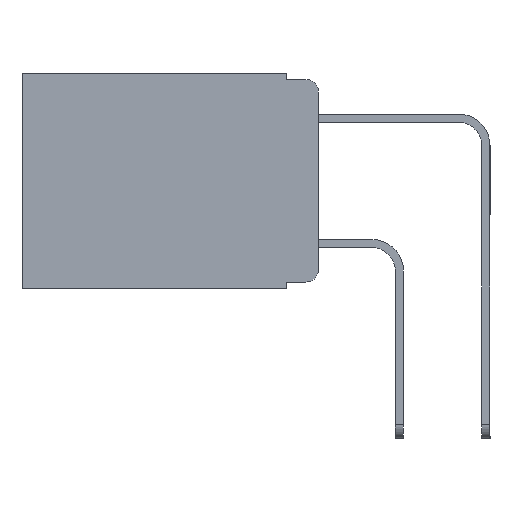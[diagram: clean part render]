
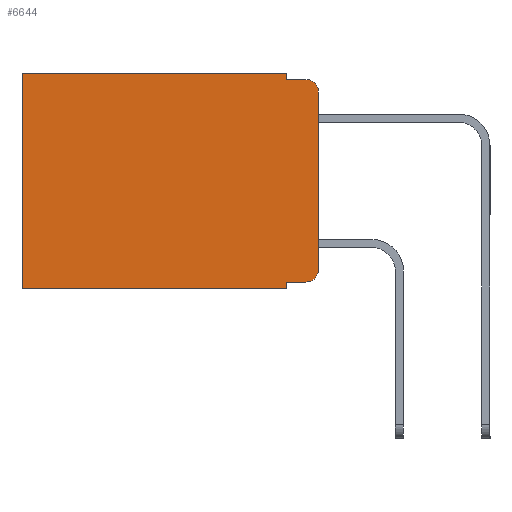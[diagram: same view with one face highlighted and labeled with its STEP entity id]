
A CAD part, left-side view. The second image highlights one B-rep face of the part: STEP entity #6644.
In plain terms, the highlighted planar face has unit normal (-1, 0, 0).
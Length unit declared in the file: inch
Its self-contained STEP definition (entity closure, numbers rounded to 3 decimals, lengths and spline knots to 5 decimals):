
#72 = ORIENTED_EDGE ( 'NONE', *, *, #3603, .T. ) ;
#216 = CARTESIAN_POINT ( 'NONE',  ( 0.298, 0., 0. ) ) ;
#468 = AXIS2_PLACEMENT_3D ( 'NONE', #3854, #10732, #11676 ) ;
#496 = DIRECTION ( 'NONE',  ( 0., 1., 0. ) ) ;
#576 = CARTESIAN_POINT ( 'NONE',  ( 0.298, 0.051, 0. ) ) ;
#677 = CARTESIAN_POINT ( 'NONE',  ( 0.298, 0.051, -0.333 ) ) ;
#688 = AXIS2_PLACEMENT_3D ( 'NONE', #8236, #6756, #6740 ) ;
#906 = CARTESIAN_POINT ( 'NONE',  ( 0.298, 0.02, -0.01 ) ) ;
#927 = CARTESIAN_POINT ( 'NONE',  ( 0.298, 0.473, -0.343 ) ) ;
#1081 = DIRECTION ( 'NONE',  ( 0., 0., -1. ) ) ;
#1325 = ORIENTED_EDGE ( 'NONE', *, *, #8675, .T. ) ;
#1689 = ORIENTED_EDGE ( 'NONE', *, *, #1794, .F. ) ;
#1720 = VERTEX_POINT ( 'NONE', #9600 ) ;
#1772 = EDGE_CURVE ( 'NONE', #12145, #12700, #9270, .T. ) ;
#1794 = EDGE_CURVE ( 'NONE', #6048, #1720, #3552, .T. ) ;
#1948 = DIRECTION ( 'NONE',  ( 0., -1., 0. ) ) ;
#2031 = ORIENTED_EDGE ( 'NONE', *, *, #2812, .F. ) ;
#2391 = VECTOR ( 'NONE', #496, 39.37008 ) ;
#2433 = VECTOR ( 'NONE', #1948, 39.37008 ) ;
#2766 = DIRECTION ( 'NONE',  ( 0., 1., 0. ) ) ;
#2773 = CARTESIAN_POINT ( 'NONE',  ( 0.298, 0.051, 0. ) ) ;
#2812 = EDGE_CURVE ( 'NONE', #8598, #4335, #10800, .T. ) ;
#3003 = FACE_OUTER_BOUND ( 'NONE', #3454, .T. ) ;
#3037 = VECTOR ( 'NONE', #5504, 39.37008 ) ;
#3120 = ORIENTED_EDGE ( 'NONE', *, *, #8449, .T. ) ;
#3154 = VECTOR ( 'NONE', #5846, 39.37008 ) ;
#3243 = VERTEX_POINT ( 'NONE', #927 ) ;
#3283 = VERTEX_POINT ( 'NONE', #9086 ) ;
#3401 = LINE ( 'NONE', #10273, #3037 ) ;
#3454 = EDGE_LOOP ( 'NONE', ( #1689, #1325, #2031, #4684, #8053, #12683, #8339, #10476, #3120, #72 ) ) ;
#3552 = LINE ( 'NONE', #5144, #9555 ) ;
#3603 = EDGE_CURVE ( 'NONE', #3283, #1720, #11099, .T. ) ;
#3854 = CARTESIAN_POINT ( 'NONE',  ( 0.298, 0.02, -0.313 ) ) ;
#4335 = VERTEX_POINT ( 'NONE', #906 ) ;
#4684 = ORIENTED_EDGE ( 'NONE', *, *, #13018, .F. ) ;
#5044 = CARTESIAN_POINT ( 'NONE',  ( 0.298, 0., -0.343 ) ) ;
#5144 = CARTESIAN_POINT ( 'NONE',  ( 0.298, 0., 0. ) ) ;
#5160 = VERTEX_POINT ( 'NONE', #8072 ) ;
#5405 = CARTESIAN_POINT ( 'NONE',  ( 0.298, 0.051, -0.333 ) ) ;
#5504 = DIRECTION ( 'NONE',  ( 0., 0., -1. ) ) ;
#5733 = LINE ( 'NONE', #5044, #2391 ) ;
#5846 = DIRECTION ( 'NONE',  ( 0., -1., 0. ) ) ;
#6048 = VERTEX_POINT ( 'NONE', #6427 ) ;
#6081 = LINE ( 'NONE', #677, #3154 ) ;
#6217 = DIRECTION ( 'NONE',  ( 0., 0., -1. ) ) ;
#6427 = CARTESIAN_POINT ( 'NONE',  ( 0.298, 0., -0.03 ) ) ;
#6507 = EDGE_CURVE ( 'NONE', #12700, #3243, #10257, .T. ) ;
#6644 = ADVANCED_FACE ( 'NONE', ( #3003 ), #10636, .F. ) ;
#6740 = DIRECTION ( 'NONE',  ( 0., 0., -1. ) ) ;
#6756 = DIRECTION ( 'NONE',  ( 1., 0., 0. ) ) ;
#7574 = DIRECTION ( 'NONE',  ( -1., 0., 0. ) ) ;
#8045 = CARTESIAN_POINT ( 'NONE',  ( 0.298, 0.473, 0. ) ) ;
#8053 = ORIENTED_EDGE ( 'NONE', *, *, #1772, .T. ) ;
#8072 = CARTESIAN_POINT ( 'NONE',  ( 0.298, 0.051, -0.343 ) ) ;
#8102 = CARTESIAN_POINT ( 'NONE',  ( 0.298, 0.473, 0. ) ) ;
#8194 = DIRECTION ( 'NONE',  ( 0., 0., -1. ) ) ;
#8236 = CARTESIAN_POINT ( 'NONE',  ( 0.298, 0., 0. ) ) ;
#8339 = ORIENTED_EDGE ( 'NONE', *, *, #9356, .F. ) ;
#8449 = EDGE_CURVE ( 'NONE', #11117, #3283, #6081, .T. ) ;
#8598 = VERTEX_POINT ( 'NONE', #11138 ) ;
#8675 = EDGE_CURVE ( 'NONE', #6048, #4335, #11226, .T. ) ;
#8982 = VECTOR ( 'NONE', #2766, 39.37008 ) ;
#9086 = CARTESIAN_POINT ( 'NONE',  ( 0.298, 0.02, -0.333 ) ) ;
#9204 = VECTOR ( 'NONE', #6217, 39.37008 ) ;
#9270 = LINE ( 'NONE', #216, #8982 ) ;
#9356 = EDGE_CURVE ( 'NONE', #5160, #3243, #5733, .T. ) ;
#9555 = VECTOR ( 'NONE', #10891, 39.37008 ) ;
#9600 = CARTESIAN_POINT ( 'NONE',  ( 0.298, 0., -0.313 ) ) ;
#9654 = AXIS2_PLACEMENT_3D ( 'NONE', #10213, #7574, #1081 ) ;
#9674 = EDGE_CURVE ( 'NONE', #11117, #5160, #9777, .T. ) ;
#9777 = LINE ( 'NONE', #2773, #9204 ) ;
#9978 = VECTOR ( 'NONE', #8194, 39.37008 ) ;
#10213 = CARTESIAN_POINT ( 'NONE',  ( 0.298, 0.02, -0.03 ) ) ;
#10257 = LINE ( 'NONE', #8102, #9978 ) ;
#10273 = CARTESIAN_POINT ( 'NONE',  ( 0.298, 0.051, 0. ) ) ;
#10476 = ORIENTED_EDGE ( 'NONE', *, *, #9674, .F. ) ;
#10636 = PLANE ( 'NONE',  #688 ) ;
#10732 = DIRECTION ( 'NONE',  ( -1., 0., 0. ) ) ;
#10800 = LINE ( 'NONE', #11192, #2433 ) ;
#10891 = DIRECTION ( 'NONE',  ( 0., 0., -1. ) ) ;
#11099 = CIRCLE ( 'NONE', #468, 0.02 ) ;
#11117 = VERTEX_POINT ( 'NONE', #5405 ) ;
#11138 = CARTESIAN_POINT ( 'NONE',  ( 0.298, 0.051, -0.01 ) ) ;
#11192 = CARTESIAN_POINT ( 'NONE',  ( 0.298, 0.051, -0.01 ) ) ;
#11226 = CIRCLE ( 'NONE', #9654, 0.02 ) ;
#11676 = DIRECTION ( 'NONE',  ( 0., 0., -1. ) ) ;
#12145 = VERTEX_POINT ( 'NONE', #576 ) ;
#12683 = ORIENTED_EDGE ( 'NONE', *, *, #6507, .T. ) ;
#12700 = VERTEX_POINT ( 'NONE', #8045 ) ;
#13018 = EDGE_CURVE ( 'NONE', #12145, #8598, #3401, .T. ) ;
